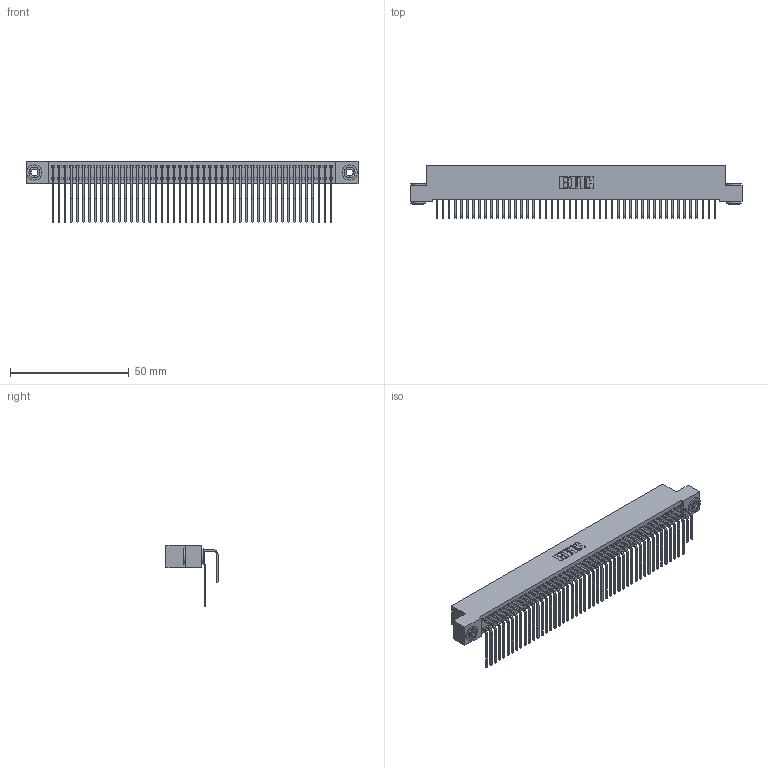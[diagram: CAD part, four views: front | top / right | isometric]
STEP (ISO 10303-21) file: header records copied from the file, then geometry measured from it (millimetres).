
FILE_DESCRIPTION (( 'STEP AP203' ), '1' );
FILE_NAME ('392-094-558-203.STEP', '2018-08-18T09:17:49', ( '' ), ( '' ), 'SwSTEP 2.0', 'SolidWorks 2016', '' );
FILE_SCHEMA (( 'CONFIG_CONTROL_DESIGN' ));
Length unit declared in the file: inch
Products named in the file (5): 342 Part_.156 TH; 345-292-001_558 559 Tail - 1; 345-292-001_558 Tail - 2; 342-250-002_345-250-002-102; 392-094-558-203
Assembly tree (97 placements, depth 2):
  392-094-558-203
    342 Part_.156 TH
    345-292-001_558 559 Tail - 1  x47
    345-292-001_558 Tail - 2  x47
    342-250-002_345-250-002-102  x2
Bounding box: 139.7 x 21.91 x 25.78 mm (x, y, z)
Volume: 13140.8 mm3; surface area: 24180.2 mm2
Topology: 97 solids, 97 shells, 5224 faces, 15509 edges, 10210 vertices
Faces by surface type: plane 3648, cylinder 1568, cone 8
Entity records: 31892 total; most frequent: CARTESIAN_POINT 5304, ORIENTED_EDGE 5182, DIRECTION 4537, EDGE_CURVE 2591, LINE 2399, VECTOR 2399, VERTEX_POINT 1722, AXIS2_PLACEMENT_3D 1069
